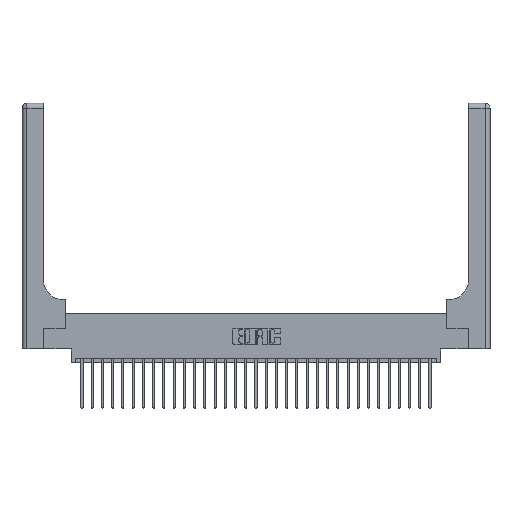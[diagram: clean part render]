
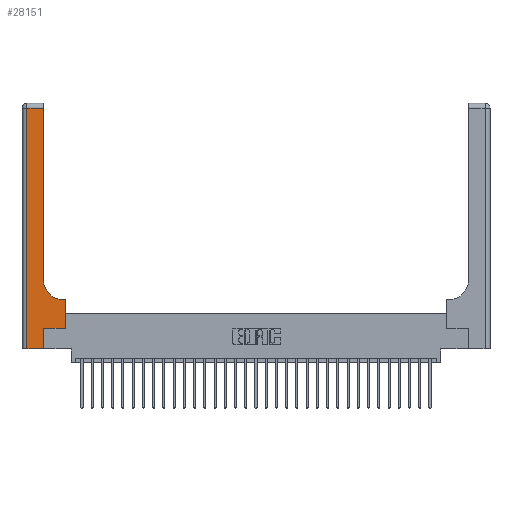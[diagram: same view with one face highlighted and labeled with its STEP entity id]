
A CAD part, top view. The second image highlights one B-rep face of the part: STEP entity #28151.
In plain terms, the highlighted planar face has unit normal (0, 0, 1).
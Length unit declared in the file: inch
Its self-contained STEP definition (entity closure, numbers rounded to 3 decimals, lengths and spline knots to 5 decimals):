
#292 = VECTOR ( 'NONE', #22010, 39.37008 ) ;
#619 = ORIENTED_EDGE ( 'NONE', *, *, #2417, .T. ) ;
#673 = VECTOR ( 'NONE', #18529, 39.37008 ) ;
#779 = CARTESIAN_POINT ( 'NONE',  ( 0.51, 0.85, 0.37 ) ) ;
#812 = LINE ( 'NONE', #21801, #23385 ) ;
#978 = VERTEX_POINT ( 'NONE', #16810 ) ;
#1693 = CARTESIAN_POINT ( 'NONE',  ( 0.06, 3., 0.37 ) ) ;
#1767 = VECTOR ( 'NONE', #8751, 39.37008 ) ;
#1834 = ORIENTED_EDGE ( 'NONE', *, *, #15418, .T. ) ;
#1995 = EDGE_CURVE ( 'NONE', #11431, #3072, #11307, .T. ) ;
#2163 = EDGE_CURVE ( 'NONE', #16006, #978, #19803, .T. ) ;
#2417 = EDGE_CURVE ( 'NONE', #26215, #16006, #18721, .T. ) ;
#2615 = CARTESIAN_POINT ( 'NONE',  ( 0.26, 0.85, 0.37 ) ) ;
#3057 = DIRECTION ( 'NONE',  ( 1., 0., 0. ) ) ;
#3072 = VERTEX_POINT ( 'NONE', #4849 ) ;
#3333 = ORIENTED_EDGE ( 'NONE', *, *, #10157, .T. ) ;
#4196 = CARTESIAN_POINT ( 'NONE',  ( 0.265, 0.25, 0.37 ) ) ;
#4849 = CARTESIAN_POINT ( 'NONE',  ( 0.51, 0.6, 0.37 ) ) ;
#4969 = VERTEX_POINT ( 'NONE', #7365 ) ;
#5517 = VERTEX_POINT ( 'NONE', #2615 ) ;
#5777 = ORIENTED_EDGE ( 'NONE', *, *, #1995, .T. ) ;
#6350 = CARTESIAN_POINT ( 'NONE',  ( 0., 3., 0.37 ) ) ;
#7280 = LINE ( 'NONE', #10375, #12580 ) ;
#7365 = CARTESIAN_POINT ( 'NONE',  ( 0.06, 2.94, 0.37 ) ) ;
#7874 = DIRECTION ( 'NONE',  ( -1., 0., 0. ) ) ;
#8619 = DIRECTION ( 'NONE',  ( -1., 0., 0. ) ) ;
#8751 = DIRECTION ( 'NONE',  ( 1., 0., 0. ) ) ;
#8771 = AXIS2_PLACEMENT_3D ( 'NONE', #779, #16579, #3057 ) ;
#8948 = VECTOR ( 'NONE', #22347, 39.37008 ) ;
#9382 = CARTESIAN_POINT ( 'NONE',  ( 0.265, 0., 0.37 ) ) ;
#9549 = VERTEX_POINT ( 'NONE', #20238 ) ;
#10114 = AXIS2_PLACEMENT_3D ( 'NONE', #6350, #22121, #8619 ) ;
#10157 = EDGE_CURVE ( 'NONE', #978, #11431, #20943, .T. ) ;
#10375 = CARTESIAN_POINT ( 'NONE',  ( 0., 0., 0.37 ) ) ;
#10726 = EDGE_CURVE ( 'NONE', #5517, #22276, #18822, .T. ) ;
#11307 = LINE ( 'NONE', #23621, #16599 ) ;
#11431 = VERTEX_POINT ( 'NONE', #21452 ) ;
#12277 = LINE ( 'NONE', #1693, #292 ) ;
#12580 = VECTOR ( 'NONE', #26087, 39.37008 ) ;
#13288 = ORIENTED_EDGE ( 'NONE', *, *, #18479, .T. ) ;
#14154 = ORIENTED_EDGE ( 'NONE', *, *, #2163, .T. ) ;
#14378 = DIRECTION ( 'NONE',  ( 0., 1., 0. ) ) ;
#14395 = ORIENTED_EDGE ( 'NONE', *, *, #21468, .T. ) ;
#14739 = EDGE_LOOP ( 'NONE', ( #26994, #13288, #14395, #18766, #619, #14154, #3333, #5777, #1834 ) ) ;
#15418 = EDGE_CURVE ( 'NONE', #3072, #5517, #24610, .T. ) ;
#16006 = VERTEX_POINT ( 'NONE', #16769 ) ;
#16579 = DIRECTION ( 'NONE',  ( 0., 0., -1. ) ) ;
#16599 = VECTOR ( 'NONE', #7874, 39.37008 ) ;
#16602 = FACE_OUTER_BOUND ( 'NONE', #14739, .T. ) ;
#16769 = CARTESIAN_POINT ( 'NONE',  ( 0.265, 0.25, 0.37 ) ) ;
#16810 = CARTESIAN_POINT ( 'NONE',  ( 0.528, 0.25, 0.37 ) ) ;
#18479 = EDGE_CURVE ( 'NONE', #22276, #4969, #812, .T. ) ;
#18529 = DIRECTION ( 'NONE',  ( 0., 1., 0. ) ) ;
#18721 = LINE ( 'NONE', #27413, #673 ) ;
#18766 = ORIENTED_EDGE ( 'NONE', *, *, #23400, .T. ) ;
#18822 = LINE ( 'NONE', #25582, #24057 ) ;
#19803 = LINE ( 'NONE', #4196, #1767 ) ;
#20238 = CARTESIAN_POINT ( 'NONE',  ( 0.06, 0., 0.37 ) ) ;
#20943 = LINE ( 'NONE', #26743, #8948 ) ;
#21452 = CARTESIAN_POINT ( 'NONE',  ( 0.528, 0.6, 0.37 ) ) ;
#21468 = EDGE_CURVE ( 'NONE', #4969, #9549, #12277, .T. ) ;
#21801 = CARTESIAN_POINT ( 'NONE',  ( 0., 2.94, 0.37 ) ) ;
#22010 = DIRECTION ( 'NONE',  ( 0., -1., 0. ) ) ;
#22121 = DIRECTION ( 'NONE',  ( 0., 0., -1. ) ) ;
#22276 = VERTEX_POINT ( 'NONE', #25956 ) ;
#22347 = DIRECTION ( 'NONE',  ( 0., 1., 0. ) ) ;
#23385 = VECTOR ( 'NONE', #26289, 39.37008 ) ;
#23400 = EDGE_CURVE ( 'NONE', #9549, #26215, #7280, .T. ) ;
#23621 = CARTESIAN_POINT ( 'NONE',  ( 0.26, 0.6, 0.37 ) ) ;
#24057 = VECTOR ( 'NONE', #14378, 39.37008 ) ;
#24258 = PLANE ( 'NONE',  #10114 ) ;
#24610 = CIRCLE ( 'NONE', #8771, 0.25 ) ;
#25582 = CARTESIAN_POINT ( 'NONE',  ( 0.26, 3., 0.37 ) ) ;
#25956 = CARTESIAN_POINT ( 'NONE',  ( 0.26, 2.94, 0.37 ) ) ;
#26087 = DIRECTION ( 'NONE',  ( 1., 0., 0. ) ) ;
#26215 = VERTEX_POINT ( 'NONE', #9382 ) ;
#26289 = DIRECTION ( 'NONE',  ( -1., 0., 0. ) ) ;
#26743 = CARTESIAN_POINT ( 'NONE',  ( 0.528, 0.25, 0.37 ) ) ;
#26994 = ORIENTED_EDGE ( 'NONE', *, *, #10726, .T. ) ;
#27413 = CARTESIAN_POINT ( 'NONE',  ( 0.265, 0., 0.37 ) ) ;
#28151 = ADVANCED_FACE ( 'NONE', ( #16602 ), #24258, .F. ) ;
